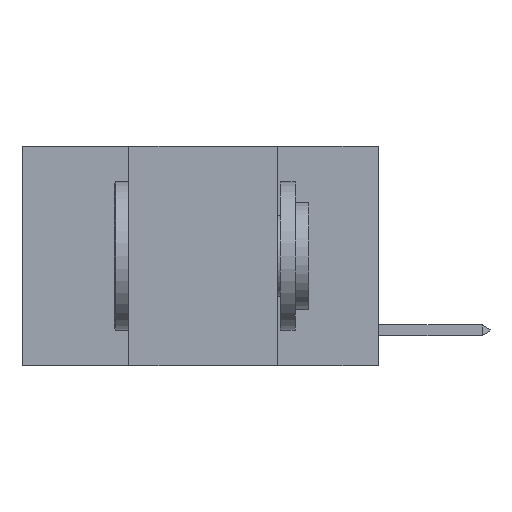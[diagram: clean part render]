
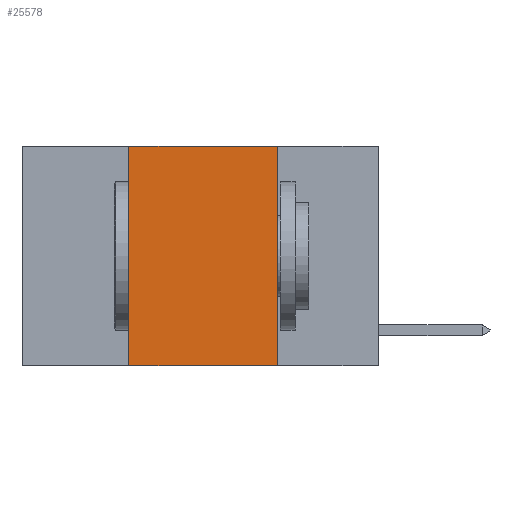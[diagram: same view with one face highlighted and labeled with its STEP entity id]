
A CAD part, left-side view. The second image highlights one B-rep face of the part: STEP entity #25578.
In plain terms, the highlighted planar face has unit normal (-1, 0, 0).
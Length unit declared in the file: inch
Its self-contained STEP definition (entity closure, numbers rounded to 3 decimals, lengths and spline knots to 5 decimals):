
#1540 = VECTOR ( 'NONE', #16460, 39.37008 ) ;
#1891 = ORIENTED_EDGE ( 'NONE', *, *, #11122, .F. ) ;
#2681 = LINE ( 'NONE', #15658, #12782 ) ;
#3891 = DIRECTION ( 'NONE',  ( 0., -1., 0. ) ) ;
#4380 = VERTEX_POINT ( 'NONE', #14235 ) ;
#4439 = EDGE_LOOP ( 'NONE', ( #16963, #14349, #1891, #17909 ) ) ;
#4787 = VECTOR ( 'NONE', #17104, 39.37008 ) ;
#4991 = EDGE_CURVE ( 'NONE', #15101, #27406, #20568, .T. ) ;
#7753 = FACE_OUTER_BOUND ( 'NONE', #4439, .T. ) ;
#8564 = EDGE_CURVE ( 'NONE', #10489, #15101, #2681, .T. ) ;
#10489 = VERTEX_POINT ( 'NONE', #29771 ) ;
#10813 = AXIS2_PLACEMENT_3D ( 'NONE', #18767, #28256, #23169 ) ;
#11122 = EDGE_CURVE ( 'NONE', #4380, #10489, #23846, .T. ) ;
#11594 = PLANE ( 'NONE',  #10813 ) ;
#12782 = VECTOR ( 'NONE', #3891, 39.37008 ) ;
#14057 = CARTESIAN_POINT ( 'NONE',  ( 0., 0.17, 0. ) ) ;
#14235 = CARTESIAN_POINT ( 'NONE',  ( 0., 0.42, -0.37 ) ) ;
#14349 = ORIENTED_EDGE ( 'NONE', *, *, #8564, .F. ) ;
#15101 = VERTEX_POINT ( 'NONE', #30878 ) ;
#15658 = CARTESIAN_POINT ( 'NONE',  ( 0., 0.6, 0. ) ) ;
#16460 = DIRECTION ( 'NONE',  ( 0., 0., -1. ) ) ;
#16963 = ORIENTED_EDGE ( 'NONE', *, *, #4991, .F. ) ;
#17104 = DIRECTION ( 'NONE',  ( 0., 0., 1. ) ) ;
#17569 = EDGE_CURVE ( 'NONE', #4380, #27406, #23285, .T. ) ;
#17909 = ORIENTED_EDGE ( 'NONE', *, *, #17569, .T. ) ;
#18767 = CARTESIAN_POINT ( 'NONE',  ( 0., 0.6, 0. ) ) ;
#18832 = CARTESIAN_POINT ( 'NONE',  ( 0., 0.17, -0.37 ) ) ;
#19137 = DIRECTION ( 'NONE',  ( 0., -1., 0. ) ) ;
#20568 = LINE ( 'NONE', #14057, #1540 ) ;
#23169 = DIRECTION ( 'NONE',  ( 0., 0., -1. ) ) ;
#23285 = LINE ( 'NONE', #26019, #29574 ) ;
#23846 = LINE ( 'NONE', #26372, #4787 ) ;
#25578 = ADVANCED_FACE ( 'NONE', ( #7753 ), #11594, .F. ) ;
#26019 = CARTESIAN_POINT ( 'NONE',  ( 0., 0.6, -0.37 ) ) ;
#26372 = CARTESIAN_POINT ( 'NONE',  ( 0., 0.42, 0. ) ) ;
#27406 = VERTEX_POINT ( 'NONE', #18832 ) ;
#28256 = DIRECTION ( 'NONE',  ( 1., 0., 0. ) ) ;
#29574 = VECTOR ( 'NONE', #19137, 39.37008 ) ;
#29771 = CARTESIAN_POINT ( 'NONE',  ( 0., 0.42, 0. ) ) ;
#30878 = CARTESIAN_POINT ( 'NONE',  ( 0., 0.17, 0. ) ) ;
